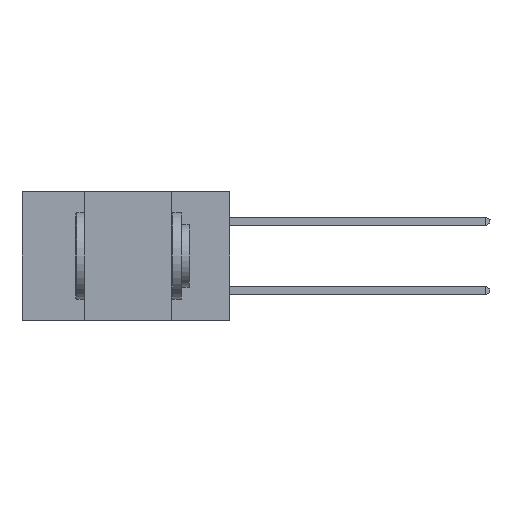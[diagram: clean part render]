
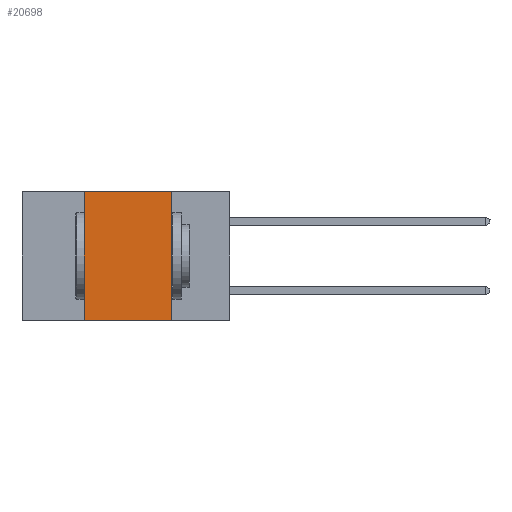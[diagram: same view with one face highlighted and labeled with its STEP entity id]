
A CAD part, left-side view. The second image highlights one B-rep face of the part: STEP entity #20698.
In plain terms, the highlighted planar face has unit normal (-1, 0, 0).
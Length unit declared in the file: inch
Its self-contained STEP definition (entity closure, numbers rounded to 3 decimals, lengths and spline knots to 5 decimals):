
#142 = LINE ( 'NONE', #18035, #13549 ) ;
#198 = ORIENTED_EDGE ( 'NONE', *, *, #5626, .F. ) ;
#509 = LINE ( 'NONE', #4056, #879 ) ;
#879 = VECTOR ( 'NONE', #9467, 39.37008 ) ;
#2816 = ORIENTED_EDGE ( 'NONE', *, *, #13317, .F. ) ;
#3102 = VECTOR ( 'NONE', #15022, 39.37008 ) ;
#3634 = DIRECTION ( 'NONE',  ( 1., 0., 0. ) ) ;
#4056 = CARTESIAN_POINT ( 'NONE',  ( 0., 0.6, -0.37 ) ) ;
#5149 = VERTEX_POINT ( 'NONE', #11541 ) ;
#5417 = CARTESIAN_POINT ( 'NONE',  ( 0., 0.6, 0. ) ) ;
#5626 = EDGE_CURVE ( 'NONE', #14931, #22768, #8895, .T. ) ;
#5758 = EDGE_CURVE ( 'NONE', #14931, #20568, #509, .T. ) ;
#7895 = CARTESIAN_POINT ( 'NONE',  ( 0., 0.17, -0.37 ) ) ;
#7899 = CARTESIAN_POINT ( 'NONE',  ( 0., 0.42, -0.37 ) ) ;
#8895 = LINE ( 'NONE', #18051, #14011 ) ;
#9467 = DIRECTION ( 'NONE',  ( 0., -1., 0. ) ) ;
#9632 = CARTESIAN_POINT ( 'NONE',  ( 0., 0.17, -0.37 ) ) ;
#10375 = AXIS2_PLACEMENT_3D ( 'NONE', #5417, #3634, #10799 ) ;
#10799 = DIRECTION ( 'NONE',  ( 0., 0., -1. ) ) ;
#10823 = EDGE_CURVE ( 'NONE', #22768, #5149, #142, .T. ) ;
#11202 = DIRECTION ( 'NONE',  ( 0., -1., 0. ) ) ;
#11541 = CARTESIAN_POINT ( 'NONE',  ( 0., 0.17, 0. ) ) ;
#12736 = ORIENTED_EDGE ( 'NONE', *, *, #5758, .T. ) ;
#13317 = EDGE_CURVE ( 'NONE', #5149, #20568, #18564, .T. ) ;
#13549 = VECTOR ( 'NONE', #11202, 39.37008 ) ;
#14011 = VECTOR ( 'NONE', #16054, 39.37008 ) ;
#14325 = FACE_OUTER_BOUND ( 'NONE', #20466, .T. ) ;
#14931 = VERTEX_POINT ( 'NONE', #7899 ) ;
#15022 = DIRECTION ( 'NONE',  ( 0., 0., -1. ) ) ;
#15785 = ORIENTED_EDGE ( 'NONE', *, *, #10823, .F. ) ;
#16054 = DIRECTION ( 'NONE',  ( 0., 0., 1. ) ) ;
#18035 = CARTESIAN_POINT ( 'NONE',  ( 0., 0.6, 0. ) ) ;
#18051 = CARTESIAN_POINT ( 'NONE',  ( 0., 0.42, -0.37 ) ) ;
#18074 = CARTESIAN_POINT ( 'NONE',  ( 0., 0.42, 0. ) ) ;
#18564 = LINE ( 'NONE', #9632, #3102 ) ;
#20466 = EDGE_LOOP ( 'NONE', ( #2816, #15785, #198, #12736 ) ) ;
#20568 = VERTEX_POINT ( 'NONE', #7895 ) ;
#20698 = ADVANCED_FACE ( 'NONE', ( #14325 ), #21504, .F. ) ;
#21504 = PLANE ( 'NONE',  #10375 ) ;
#22768 = VERTEX_POINT ( 'NONE', #18074 ) ;
